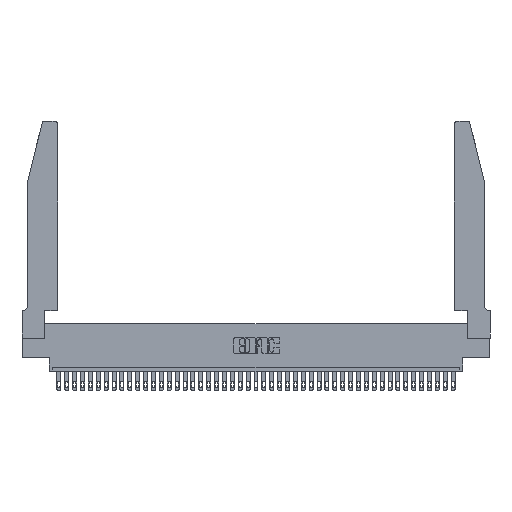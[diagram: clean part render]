
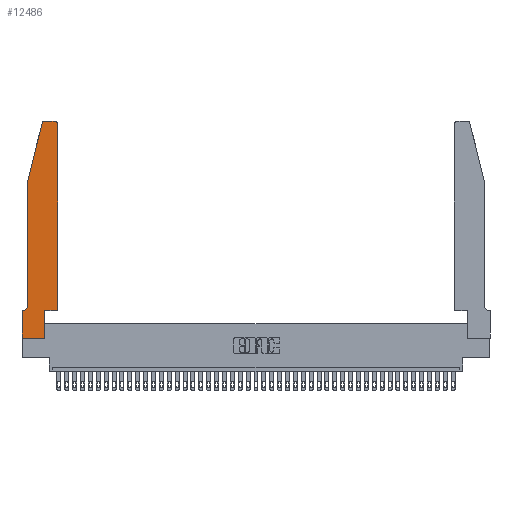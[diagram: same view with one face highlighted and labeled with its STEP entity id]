
A CAD part, top view. The second image highlights one B-rep face of the part: STEP entity #12486.
In plain terms, the highlighted planar face has unit normal (0, 0, 1).
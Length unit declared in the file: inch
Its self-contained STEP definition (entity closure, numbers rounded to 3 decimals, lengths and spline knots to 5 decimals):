
#83 = CARTESIAN_POINT ( 'NONE',  ( 0.25487, 2.72718, 0.37 ) ) ;
#637 = EDGE_CURVE ( 'NONE', #8638, #4082, #21514, .T. ) ;
#793 = CIRCLE ( 'NONE', #27587, 0.07 ) ;
#1046 = ORIENTED_EDGE ( 'NONE', *, *, #2092, .T. ) ;
#1799 = CARTESIAN_POINT ( 'NONE',  ( 0., 0.35, 0.37 ) ) ;
#2092 = EDGE_CURVE ( 'NONE', #21739, #26627, #18783, .T. ) ;
#2435 = ORIENTED_EDGE ( 'NONE', *, *, #5848, .T. ) ;
#2559 = ORIENTED_EDGE ( 'NONE', *, *, #13565, .T. ) ;
#2651 = DIRECTION ( 'NONE',  ( 1., 0., 0. ) ) ;
#2854 = DIRECTION ( 'NONE',  ( 0., -1., 0. ) ) ;
#2876 = DIRECTION ( 'NONE',  ( -1., 0., 0. ) ) ;
#4082 = VERTEX_POINT ( 'NONE', #22155 ) ;
#4281 = LINE ( 'NONE', #6291, #40798 ) ;
#4332 = VECTOR ( 'NONE', #19460, 39.37008 ) ;
#4716 = LINE ( 'NONE', #31152, #19419 ) ;
#5848 = EDGE_CURVE ( 'NONE', #26627, #31704, #16956, .T. ) ;
#6291 = CARTESIAN_POINT ( 'NONE',  ( 0.2605, 2.75, 0.37 ) ) ;
#6577 = EDGE_CURVE ( 'NONE', #39346, #19845, #4716, .T. ) ;
#6821 = EDGE_CURVE ( 'NONE', #20259, #8638, #18915, .T. ) ;
#7361 = VECTOR ( 'NONE', #21365, 39.37008 ) ;
#7634 = DIRECTION ( 'NONE',  ( -1., 0., 0. ) ) ;
#7930 = CIRCLE ( 'NONE', #14655, 0.03 ) ;
#8228 = CARTESIAN_POINT ( 'NONE',  ( 0.0055, 0.42, 0.37 ) ) ;
#8377 = CARTESIAN_POINT ( 'NONE',  ( 0.0755, 0.42, 0.37 ) ) ;
#8585 = CARTESIAN_POINT ( 'NONE',  ( 0., 0.35, 0.37 ) ) ;
#8638 = VERTEX_POINT ( 'NONE', #36934 ) ;
#8951 = LINE ( 'NONE', #41131, #38278 ) ;
#9032 = DIRECTION ( 'NONE',  ( 0., 0., 1. ) ) ;
#9413 = CARTESIAN_POINT ( 'NONE',  ( 0.2865, 0., 0.37 ) ) ;
#10182 = VERTEX_POINT ( 'NONE', #40119 ) ;
#12486 = ADVANCED_FACE ( 'NONE', ( #35820 ), #17599, .T. ) ;
#12646 = AXIS2_PLACEMENT_3D ( 'NONE', #8585, #15077, #20986 ) ;
#13308 = ORIENTED_EDGE ( 'NONE', *, *, #6577, .T. ) ;
#13565 = EDGE_CURVE ( 'NONE', #10182, #21739, #4281, .T. ) ;
#14655 = AXIS2_PLACEMENT_3D ( 'NONE', #22319, #35104, #38616 ) ;
#15077 = DIRECTION ( 'NONE',  ( 0., 0., 1. ) ) ;
#15628 = CARTESIAN_POINT ( 'NONE',  ( 0.4505, 0.35, 0.37 ) ) ;
#16136 = ORIENTED_EDGE ( 'NONE', *, *, #637, .T. ) ;
#16230 = CARTESIAN_POINT ( 'NONE',  ( 0., 0., 0.37 ) ) ;
#16275 = EDGE_CURVE ( 'NONE', #4082, #10182, #7930, .T. ) ;
#16420 = DIRECTION ( 'NONE',  ( 1., 0., 0. ) ) ;
#16489 = VECTOR ( 'NONE', #28458, 39.37008 ) ;
#16621 = CARTESIAN_POINT ( 'NONE',  ( 0.0055, 0.35, 0.37 ) ) ;
#16956 = LINE ( 'NONE', #17840, #7361 ) ;
#17023 = EDGE_CURVE ( 'NONE', #27141, #20259, #8951, .T. ) ;
#17112 = CARTESIAN_POINT ( 'NONE',  ( 0., 0., 0.37 ) ) ;
#17328 = EDGE_CURVE ( 'NONE', #31704, #25871, #34721, .T. ) ;
#17599 = PLANE ( 'NONE',  #12646 ) ;
#17840 = CARTESIAN_POINT ( 'NONE',  ( 0.0755, 2., 0.37 ) ) ;
#18562 = CARTESIAN_POINT ( 'NONE',  ( 0.0755, 2., 0.37 ) ) ;
#18783 = CIRCLE ( 'NONE', #35966, 0.03 ) ;
#18915 = LINE ( 'NONE', #26009, #21395 ) ;
#19419 = VECTOR ( 'NONE', #27602, 39.37008 ) ;
#19460 = DIRECTION ( 'NONE',  ( 1., 0., 0. ) ) ;
#19845 = VERTEX_POINT ( 'NONE', #17112 ) ;
#19940 = VECTOR ( 'NONE', #2854, 39.37008 ) ;
#20259 = VERTEX_POINT ( 'NONE', #38210 ) ;
#20650 = EDGE_LOOP ( 'NONE', ( #2559, #1046, #2435, #22156, #25701, #37055, #13308, #23315, #22228, #31576, #16136, #33042 ) ) ;
#20986 = DIRECTION ( 'NONE',  ( 1., 0., 0. ) ) ;
#21079 = DIRECTION ( 'NONE',  ( -1., 0., 0. ) ) ;
#21350 = VECTOR ( 'NONE', #21079, 39.37008 ) ;
#21365 = DIRECTION ( 'NONE',  ( -0.239, -0.971, 0. ) ) ;
#21395 = VECTOR ( 'NONE', #16420, 39.37008 ) ;
#21514 = LINE ( 'NONE', #15628, #16489 ) ;
#21739 = VERTEX_POINT ( 'NONE', #28699 ) ;
#22155 = CARTESIAN_POINT ( 'NONE',  ( 0.4505, 2.72, 0.37 ) ) ;
#22156 = ORIENTED_EDGE ( 'NONE', *, *, #17328, .T. ) ;
#22228 = ORIENTED_EDGE ( 'NONE', *, *, #17023, .T. ) ;
#22319 = CARTESIAN_POINT ( 'NONE',  ( 0.4205, 2.72, 0.37 ) ) ;
#23131 = EDGE_CURVE ( 'NONE', #26722, #39346, #39065, .T. ) ;
#23315 = ORIENTED_EDGE ( 'NONE', *, *, #26674, .T. ) ;
#24765 = CARTESIAN_POINT ( 'NONE',  ( 0.0755, 2., 0.37 ) ) ;
#25126 = DIRECTION ( 'NONE',  ( 0., 1., 0. ) ) ;
#25128 = LINE ( 'NONE', #16230, #4332 ) ;
#25701 = ORIENTED_EDGE ( 'NONE', *, *, #25798, .T. ) ;
#25798 = EDGE_CURVE ( 'NONE', #25871, #26722, #793, .T. ) ;
#25871 = VERTEX_POINT ( 'NONE', #8377 ) ;
#26009 = CARTESIAN_POINT ( 'NONE',  ( 0.4505, 0.35, 0.37 ) ) ;
#26627 = VERTEX_POINT ( 'NONE', #83 ) ;
#26674 = EDGE_CURVE ( 'NONE', #19845, #27141, #25128, .T. ) ;
#26722 = VERTEX_POINT ( 'NONE', #16621 ) ;
#27136 = CARTESIAN_POINT ( 'NONE',  ( 0.0755, 0.35, 0.37 ) ) ;
#27141 = VERTEX_POINT ( 'NONE', #9413 ) ;
#27587 = AXIS2_PLACEMENT_3D ( 'NONE', #8228, #37062, #7634 ) ;
#27602 = DIRECTION ( 'NONE',  ( 0., -1., 0. ) ) ;
#28458 = DIRECTION ( 'NONE',  ( 0., 1., 0. ) ) ;
#28699 = CARTESIAN_POINT ( 'NONE',  ( 0.284, 2.75, 0.37 ) ) ;
#31152 = CARTESIAN_POINT ( 'NONE',  ( 0., 0., 0.37 ) ) ;
#31576 = ORIENTED_EDGE ( 'NONE', *, *, #6821, .T. ) ;
#31704 = VERTEX_POINT ( 'NONE', #24765 ) ;
#33042 = ORIENTED_EDGE ( 'NONE', *, *, #16275, .T. ) ;
#34721 = LINE ( 'NONE', #18562, #19940 ) ;
#35104 = DIRECTION ( 'NONE',  ( 0., 0., 1. ) ) ;
#35820 = FACE_OUTER_BOUND ( 'NONE', #20650, .T. ) ;
#35966 = AXIS2_PLACEMENT_3D ( 'NONE', #38707, #9032, #2651 ) ;
#36934 = CARTESIAN_POINT ( 'NONE',  ( 0.4505, 0.35, 0.37 ) ) ;
#37055 = ORIENTED_EDGE ( 'NONE', *, *, #23131, .T. ) ;
#37062 = DIRECTION ( 'NONE',  ( 0., 0., -1. ) ) ;
#38210 = CARTESIAN_POINT ( 'NONE',  ( 0.2865, 0.35, 0.37 ) ) ;
#38278 = VECTOR ( 'NONE', #25126, 39.37008 ) ;
#38616 = DIRECTION ( 'NONE',  ( 1., 0., 0. ) ) ;
#38707 = CARTESIAN_POINT ( 'NONE',  ( 0.284, 2.72, 0.37 ) ) ;
#39065 = LINE ( 'NONE', #27136, #21350 ) ;
#39346 = VERTEX_POINT ( 'NONE', #1799 ) ;
#40119 = CARTESIAN_POINT ( 'NONE',  ( 0.4205, 2.75, 0.37 ) ) ;
#40798 = VECTOR ( 'NONE', #2876, 39.37008 ) ;
#41131 = CARTESIAN_POINT ( 'NONE',  ( 0.2865, 0.35, 0.37 ) ) ;
